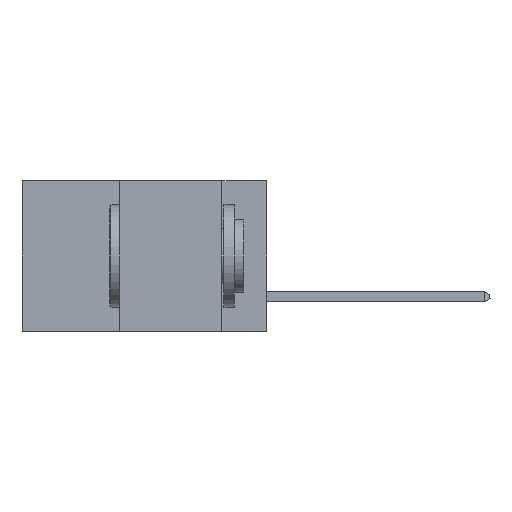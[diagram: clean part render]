
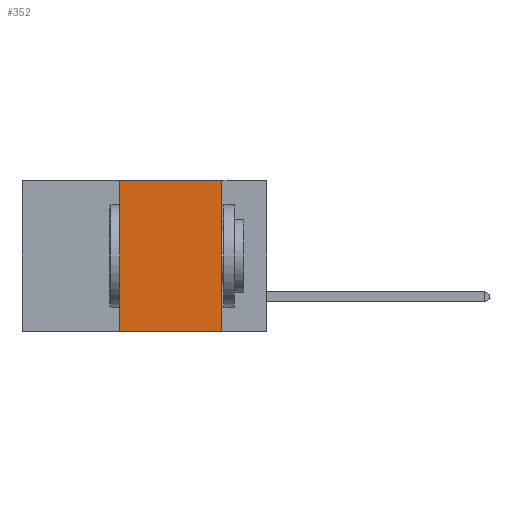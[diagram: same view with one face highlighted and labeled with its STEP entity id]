
A CAD part, left-side view. The second image highlights one B-rep face of the part: STEP entity #352.
In plain terms, the highlighted planar face has unit normal (-1, 0, 0).
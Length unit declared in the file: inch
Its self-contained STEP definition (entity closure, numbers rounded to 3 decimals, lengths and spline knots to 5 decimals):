
#352 = ADVANCED_FACE ( 'NONE', ( #21436 ), #24862, .F. ) ;
#439 = CARTESIAN_POINT ( 'NONE',  ( 0., 0.6, 0. ) ) ;
#866 = LINE ( 'NONE', #8728, #12582 ) ;
#2993 = EDGE_LOOP ( 'NONE', ( #13340, #28195, #19813, #20568 ) ) ;
#3324 = AXIS2_PLACEMENT_3D ( 'NONE', #439, #32533, #4346 ) ;
#4346 = DIRECTION ( 'NONE',  ( 0., 0., -1. ) ) ;
#5145 = EDGE_CURVE ( 'NONE', #32464, #26475, #16885, .T. ) ;
#8728 = CARTESIAN_POINT ( 'NONE',  ( 0., 0.6, -0.37 ) ) ;
#9739 = CARTESIAN_POINT ( 'NONE',  ( 0., 0.36, 0. ) ) ;
#10704 = EDGE_CURVE ( 'NONE', #44531, #32464, #29063, .T. ) ;
#12582 = VECTOR ( 'NONE', #16044, 39.37008 ) ;
#12720 = DIRECTION ( 'NONE',  ( 0., 0., 1. ) ) ;
#13340 = ORIENTED_EDGE ( 'NONE', *, *, #18541, .F. ) ;
#15773 = CARTESIAN_POINT ( 'NONE',  ( 0., 0.6, 0. ) ) ;
#16044 = DIRECTION ( 'NONE',  ( 0., -1., 0. ) ) ;
#16885 = LINE ( 'NONE', #15773, #33431 ) ;
#16966 = VECTOR ( 'NONE', #12720, 39.37008 ) ;
#17866 = EDGE_CURVE ( 'NONE', #44531, #40263, #866, .T. ) ;
#18541 = EDGE_CURVE ( 'NONE', #26475, #40263, #30321, .T. ) ;
#19225 = VECTOR ( 'NONE', #42227, 39.37008 ) ;
#19703 = CARTESIAN_POINT ( 'NONE',  ( 0., 0.36, 0. ) ) ;
#19813 = ORIENTED_EDGE ( 'NONE', *, *, #10704, .F. ) ;
#20568 = ORIENTED_EDGE ( 'NONE', *, *, #17866, .T. ) ;
#21436 = FACE_OUTER_BOUND ( 'NONE', #2993, .T. ) ;
#24862 = PLANE ( 'NONE',  #3324 ) ;
#26475 = VERTEX_POINT ( 'NONE', #29602 ) ;
#28195 = ORIENTED_EDGE ( 'NONE', *, *, #5145, .F. ) ;
#29063 = LINE ( 'NONE', #19703, #16966 ) ;
#29602 = CARTESIAN_POINT ( 'NONE',  ( 0., 0.11, 0. ) ) ;
#30321 = LINE ( 'NONE', #36959, #19225 ) ;
#32464 = VERTEX_POINT ( 'NONE', #9739 ) ;
#32533 = DIRECTION ( 'NONE',  ( 1., 0., 0. ) ) ;
#33431 = VECTOR ( 'NONE', #43509, 39.37008 ) ;
#36152 = CARTESIAN_POINT ( 'NONE',  ( 0., 0.11, -0.37 ) ) ;
#36959 = CARTESIAN_POINT ( 'NONE',  ( 0., 0.11, 0. ) ) ;
#40263 = VERTEX_POINT ( 'NONE', #36152 ) ;
#42227 = DIRECTION ( 'NONE',  ( 0., 0., -1. ) ) ;
#43509 = DIRECTION ( 'NONE',  ( 0., -1., 0. ) ) ;
#44063 = CARTESIAN_POINT ( 'NONE',  ( 0., 0.36, -0.37 ) ) ;
#44531 = VERTEX_POINT ( 'NONE', #44063 ) ;
